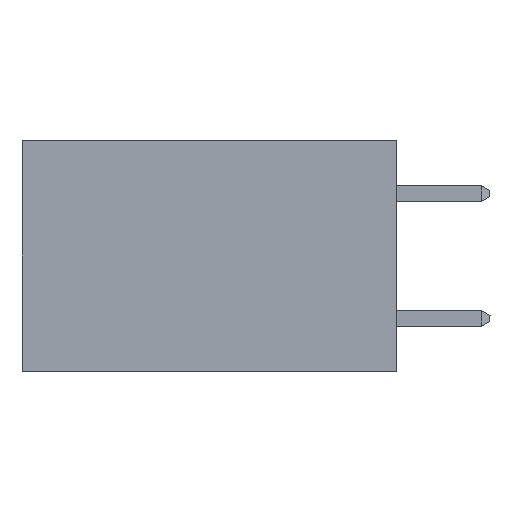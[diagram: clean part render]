
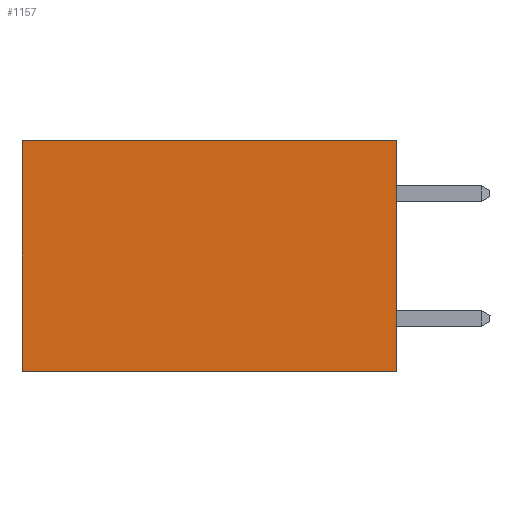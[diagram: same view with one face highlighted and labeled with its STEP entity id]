
A CAD part, left-side view. The second image highlights one B-rep face of the part: STEP entity #1157.
In plain terms, the highlighted planar face has unit normal (-1, 0, 0).
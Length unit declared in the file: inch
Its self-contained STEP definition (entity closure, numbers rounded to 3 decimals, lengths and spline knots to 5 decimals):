
#88 = VERTEX_POINT ( 'NONE', #2156 ) ;
#738 = DIRECTION ( 'NONE',  ( 1., 0., 0. ) ) ;
#920 = CARTESIAN_POINT ( 'NONE',  ( 0.298, 0., 0. ) ) ;
#945 = FACE_OUTER_BOUND ( 'NONE', #5362, .T. ) ;
#1157 = ADVANCED_FACE ( 'NONE', ( #945 ), #6745, .F. ) ;
#1187 = ORIENTED_EDGE ( 'NONE', *, *, #1261, .F. ) ;
#1261 = EDGE_CURVE ( 'NONE', #88, #3471, #7312, .T. ) ;
#1368 = CARTESIAN_POINT ( 'NONE',  ( 0.298, 0., -0.37 ) ) ;
#1634 = CARTESIAN_POINT ( 'NONE',  ( 0.298, 0.6, -0.37 ) ) ;
#1779 = EDGE_CURVE ( 'NONE', #3471, #5804, #3975, .T. ) ;
#2010 = VECTOR ( 'NONE', #9510, 39.37008 ) ;
#2110 = DIRECTION ( 'NONE',  ( 0., 1., 0. ) ) ;
#2156 = CARTESIAN_POINT ( 'NONE',  ( 0.298, 0., 0. ) ) ;
#2506 = LINE ( 'NONE', #2569, #8744 ) ;
#2569 = CARTESIAN_POINT ( 'NONE',  ( 0.298, 0., 0. ) ) ;
#2721 = AXIS2_PLACEMENT_3D ( 'NONE', #3392, #738, #3250 ) ;
#3250 = DIRECTION ( 'NONE',  ( 0., 0., -1. ) ) ;
#3392 = CARTESIAN_POINT ( 'NONE',  ( 0.298, 0., 0. ) ) ;
#3471 = VERTEX_POINT ( 'NONE', #1368 ) ;
#3576 = ORIENTED_EDGE ( 'NONE', *, *, #1779, .F. ) ;
#3632 = ORIENTED_EDGE ( 'NONE', *, *, #4041, .T. ) ;
#3975 = LINE ( 'NONE', #9019, #6365 ) ;
#4041 = EDGE_CURVE ( 'NONE', #88, #5017, #2506, .T. ) ;
#4807 = CARTESIAN_POINT ( 'NONE',  ( 0.298, 0.6, 0. ) ) ;
#4809 = VECTOR ( 'NONE', #6484, 39.37008 ) ;
#5017 = VERTEX_POINT ( 'NONE', #5890 ) ;
#5338 = LINE ( 'NONE', #4807, #4809 ) ;
#5362 = EDGE_LOOP ( 'NONE', ( #9947, #3576, #1187, #3632 ) ) ;
#5804 = VERTEX_POINT ( 'NONE', #1634 ) ;
#5890 = CARTESIAN_POINT ( 'NONE',  ( 0.298, 0.6, 0. ) ) ;
#6365 = VECTOR ( 'NONE', #2110, 39.37008 ) ;
#6484 = DIRECTION ( 'NONE',  ( 0., 0., -1. ) ) ;
#6745 = PLANE ( 'NONE',  #2721 ) ;
#7312 = LINE ( 'NONE', #920, #2010 ) ;
#8465 = DIRECTION ( 'NONE',  ( 0., 1., 0. ) ) ;
#8744 = VECTOR ( 'NONE', #8465, 39.37008 ) ;
#9019 = CARTESIAN_POINT ( 'NONE',  ( 0.298, 0., -0.37 ) ) ;
#9510 = DIRECTION ( 'NONE',  ( 0., 0., -1. ) ) ;
#9621 = EDGE_CURVE ( 'NONE', #5017, #5804, #5338, .T. ) ;
#9947 = ORIENTED_EDGE ( 'NONE', *, *, #9621, .T. ) ;
